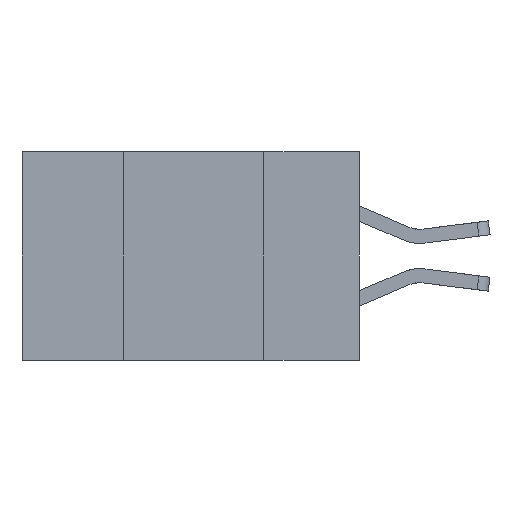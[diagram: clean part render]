
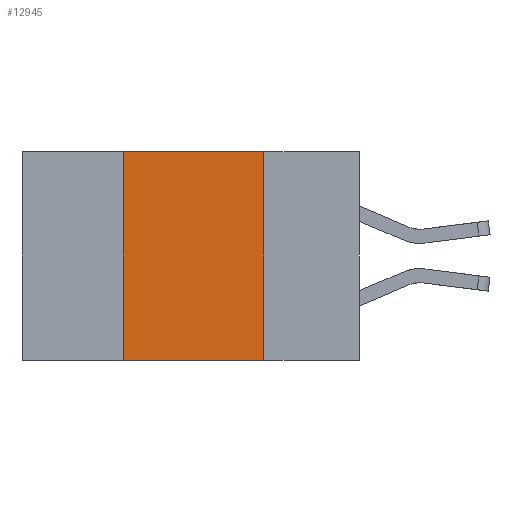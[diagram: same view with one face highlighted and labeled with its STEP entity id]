
A CAD part, left-side view. The second image highlights one B-rep face of the part: STEP entity #12945.
In plain terms, the highlighted planar face has unit normal (-1, 0, 0).
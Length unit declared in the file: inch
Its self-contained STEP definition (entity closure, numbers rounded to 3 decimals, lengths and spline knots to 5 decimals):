
#562 = EDGE_CURVE ( 'NONE', #7691, #10562, #1221, .T. ) ;
#811 = LINE ( 'NONE', #5065, #1563 ) ;
#1035 = VECTOR ( 'NONE', #12192, 39.37008 ) ;
#1221 = LINE ( 'NONE', #2267, #9780 ) ;
#1370 = VERTEX_POINT ( 'NONE', #11570 ) ;
#1563 = VECTOR ( 'NONE', #11435, 39.37008 ) ;
#1591 = ORIENTED_EDGE ( 'NONE', *, *, #11474, .F. ) ;
#1787 = CARTESIAN_POINT ( 'NONE',  ( 0., 0.17, -0.37 ) ) ;
#1963 = ORIENTED_EDGE ( 'NONE', *, *, #11853, .F. ) ;
#2267 = CARTESIAN_POINT ( 'NONE',  ( 0., 0.17, 0. ) ) ;
#2607 = CARTESIAN_POINT ( 'NONE',  ( 0., 0.42, -0.37 ) ) ;
#2707 = CARTESIAN_POINT ( 'NONE',  ( 0., 0.6, 0. ) ) ;
#2931 = CARTESIAN_POINT ( 'NONE',  ( 0., 0.6, 0. ) ) ;
#3522 = EDGE_LOOP ( 'NONE', ( #4020, #1963, #1591, #12700 ) ) ;
#3833 = DIRECTION ( 'NONE',  ( 0., -1., 0. ) ) ;
#4020 = ORIENTED_EDGE ( 'NONE', *, *, #562, .F. ) ;
#5057 = CARTESIAN_POINT ( 'NONE',  ( 0., 0.17, 0. ) ) ;
#5065 = CARTESIAN_POINT ( 'NONE',  ( 0., 0.42, 0. ) ) ;
#5486 = DIRECTION ( 'NONE',  ( 0., 0., -1. ) ) ;
#5545 = VERTEX_POINT ( 'NONE', #2607 ) ;
#5605 = DIRECTION ( 'NONE',  ( 0., 0., -1. ) ) ;
#6028 = LINE ( 'NONE', #2707, #1035 ) ;
#6965 = CARTESIAN_POINT ( 'NONE',  ( 0., 0.6, -0.37 ) ) ;
#7691 = VERTEX_POINT ( 'NONE', #5057 ) ;
#9006 = EDGE_CURVE ( 'NONE', #5545, #10562, #13325, .T. ) ;
#9314 = PLANE ( 'NONE',  #10365 ) ;
#9780 = VECTOR ( 'NONE', #5605, 39.37008 ) ;
#10365 = AXIS2_PLACEMENT_3D ( 'NONE', #2931, #11330, #5486 ) ;
#10562 = VERTEX_POINT ( 'NONE', #1787 ) ;
#11330 = DIRECTION ( 'NONE',  ( 1., 0., 0. ) ) ;
#11393 = VECTOR ( 'NONE', #3833, 39.37008 ) ;
#11435 = DIRECTION ( 'NONE',  ( 0., 0., 1. ) ) ;
#11474 = EDGE_CURVE ( 'NONE', #5545, #1370, #811, .T. ) ;
#11570 = CARTESIAN_POINT ( 'NONE',  ( 0., 0.42, 0. ) ) ;
#11853 = EDGE_CURVE ( 'NONE', #1370, #7691, #6028, .T. ) ;
#12192 = DIRECTION ( 'NONE',  ( 0., -1., 0. ) ) ;
#12549 = FACE_OUTER_BOUND ( 'NONE', #3522, .T. ) ;
#12700 = ORIENTED_EDGE ( 'NONE', *, *, #9006, .T. ) ;
#12945 = ADVANCED_FACE ( 'NONE', ( #12549 ), #9314, .F. ) ;
#13325 = LINE ( 'NONE', #6965, #11393 ) ;
